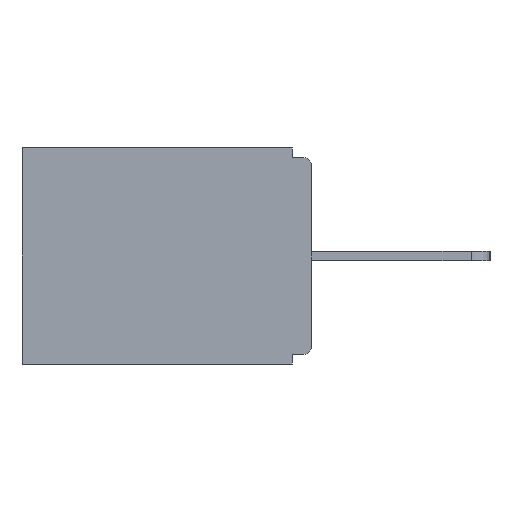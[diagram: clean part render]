
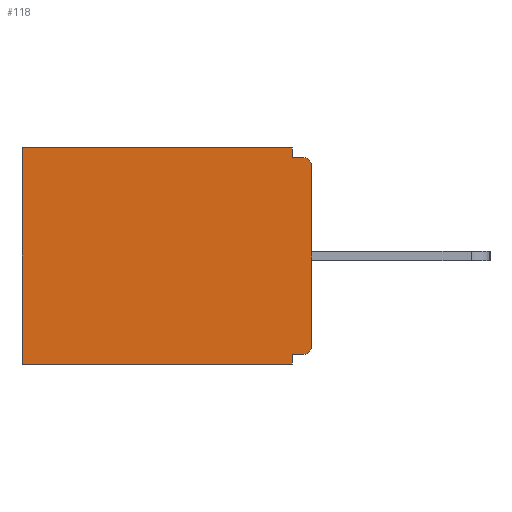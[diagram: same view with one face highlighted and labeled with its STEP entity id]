
A CAD part, left-side view. The second image highlights one B-rep face of the part: STEP entity #118.
In plain terms, the highlighted planar face has unit normal (-1, 0, 0).
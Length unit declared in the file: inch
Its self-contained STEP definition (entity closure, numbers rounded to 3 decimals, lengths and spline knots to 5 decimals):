
#29 = ORIENTED_EDGE ( 'NONE', *, *, #69, .F. ) ;
#69 = EDGE_CURVE ( 'NONE', #5602, #6535, #3409, .T. ) ;
#118 = ADVANCED_FACE ( 'NONE', ( #5495 ), #9830, .F. ) ;
#1013 = CARTESIAN_POINT ( 'NONE',  ( 0.298, 0.031, -0.343 ) ) ;
#1296 = VERTEX_POINT ( 'NONE', #2700 ) ;
#1427 = ORIENTED_EDGE ( 'NONE', *, *, #3058, .F. ) ;
#1451 = VERTEX_POINT ( 'NONE', #1707 ) ;
#1529 = ORIENTED_EDGE ( 'NONE', *, *, #13600, .T. ) ;
#1683 = CIRCLE ( 'NONE', #3444, 0.015 ) ;
#1707 = CARTESIAN_POINT ( 'NONE',  ( 0.298, 0.031, -0.343 ) ) ;
#1719 = VECTOR ( 'NONE', #12653, 39.37008 ) ;
#1757 = CARTESIAN_POINT ( 'NONE',  ( 0.298, 0.031, 0. ) ) ;
#1903 = VECTOR ( 'NONE', #17401, 39.37008 ) ;
#2360 = EDGE_CURVE ( 'NONE', #8241, #4948, #3593, .T. ) ;
#2376 = LINE ( 'NONE', #17199, #6337 ) ;
#2412 = LINE ( 'NONE', #14303, #10212 ) ;
#2489 = ORIENTED_EDGE ( 'NONE', *, *, #14761, .F. ) ;
#2700 = CARTESIAN_POINT ( 'NONE',  ( 0.298, 0.46, 0. ) ) ;
#2850 = CARTESIAN_POINT ( 'NONE',  ( 0.298, 0.015, -0.015 ) ) ;
#2875 = EDGE_CURVE ( 'NONE', #5602, #15154, #1683, .T. ) ;
#2887 = DIRECTION ( 'NONE',  ( 0., 0., -1. ) ) ;
#3058 = EDGE_CURVE ( 'NONE', #7864, #7671, #2376, .T. ) ;
#3164 = CARTESIAN_POINT ( 'NONE',  ( 0.298, 0., 0. ) ) ;
#3295 = CARTESIAN_POINT ( 'NONE',  ( 0.298, 0., 0. ) ) ;
#3409 = LINE ( 'NONE', #9230, #13443 ) ;
#3413 = EDGE_LOOP ( 'NONE', ( #5594, #10567, #1427, #1529, #5891, #2489, #17662, #15409, #12794, #29 ) ) ;
#3444 = AXIS2_PLACEMENT_3D ( 'NONE', #6610, #6570, #6550 ) ;
#3593 = LINE ( 'NONE', #6092, #17452 ) ;
#3798 = DIRECTION ( 'NONE',  ( 1., 0., 0. ) ) ;
#3959 = DIRECTION ( 'NONE',  ( 0., 1., 0. ) ) ;
#4643 = CARTESIAN_POINT ( 'NONE',  ( 0.298, 0.46, -0.343 ) ) ;
#4800 = DIRECTION ( 'NONE',  ( 0., 1., 0. ) ) ;
#4948 = VERTEX_POINT ( 'NONE', #13996 ) ;
#5204 = DIRECTION ( 'NONE',  ( 0., 0., -1. ) ) ;
#5298 = CARTESIAN_POINT ( 'NONE',  ( 0.298, 0., -0.03 ) ) ;
#5495 = FACE_OUTER_BOUND ( 'NONE', #3413, .T. ) ;
#5594 = ORIENTED_EDGE ( 'NONE', *, *, #2875, .T. ) ;
#5602 = VERTEX_POINT ( 'NONE', #5298 ) ;
#5680 = LINE ( 'NONE', #1013, #1719 ) ;
#5891 = ORIENTED_EDGE ( 'NONE', *, *, #10543, .T. ) ;
#6092 = CARTESIAN_POINT ( 'NONE',  ( 0.298, 0., -0.328 ) ) ;
#6204 = VERTEX_POINT ( 'NONE', #4643 ) ;
#6337 = VECTOR ( 'NONE', #14856, 39.37008 ) ;
#6535 = VERTEX_POINT ( 'NONE', #14258 ) ;
#6550 = DIRECTION ( 'NONE',  ( 0., 0., -1. ) ) ;
#6570 = DIRECTION ( 'NONE',  ( -1., 0., 0. ) ) ;
#6610 = CARTESIAN_POINT ( 'NONE',  ( 0.298, 0.015, -0.03 ) ) ;
#7373 = DIRECTION ( 'NONE',  ( 0., -1., 0. ) ) ;
#7671 = VERTEX_POINT ( 'NONE', #17305 ) ;
#7864 = VERTEX_POINT ( 'NONE', #1757 ) ;
#7906 = CARTESIAN_POINT ( 'NONE',  ( 0.298, 0., -0.343 ) ) ;
#8040 = LINE ( 'NONE', #9555, #11451 ) ;
#8241 = VERTEX_POINT ( 'NONE', #14052 ) ;
#9121 = EDGE_CURVE ( 'NONE', #8241, #6535, #12756, .T. ) ;
#9230 = CARTESIAN_POINT ( 'NONE',  ( 0.298, 0., 0. ) ) ;
#9555 = CARTESIAN_POINT ( 'NONE',  ( 0.298, 0.46, 0. ) ) ;
#9830 = PLANE ( 'NONE',  #15934 ) ;
#10212 = VECTOR ( 'NONE', #7373, 39.37008 ) ;
#10543 = EDGE_CURVE ( 'NONE', #1296, #6204, #8040, .T. ) ;
#10567 = ORIENTED_EDGE ( 'NONE', *, *, #17330, .F. ) ;
#11451 = VECTOR ( 'NONE', #5204, 39.37008 ) ;
#12653 = DIRECTION ( 'NONE',  ( 0., 0., -1. ) ) ;
#12756 = CIRCLE ( 'NONE', #14075, 0.015 ) ;
#12794 = ORIENTED_EDGE ( 'NONE', *, *, #9121, .T. ) ;
#12955 = LINE ( 'NONE', #7906, #1903 ) ;
#13443 = VECTOR ( 'NONE', #15652, 39.37008 ) ;
#13600 = EDGE_CURVE ( 'NONE', #7864, #1296, #18027, .T. ) ;
#13996 = CARTESIAN_POINT ( 'NONE',  ( 0.298, 0.031, -0.328 ) ) ;
#14052 = CARTESIAN_POINT ( 'NONE',  ( 0.298, 0.015, -0.328 ) ) ;
#14075 = AXIS2_PLACEMENT_3D ( 'NONE', #15311, #16979, #16953 ) ;
#14258 = CARTESIAN_POINT ( 'NONE',  ( 0.298, 0., -0.313 ) ) ;
#14303 = CARTESIAN_POINT ( 'NONE',  ( 0.298, 0., -0.015 ) ) ;
#14595 = VECTOR ( 'NONE', #4800, 39.37008 ) ;
#14761 = EDGE_CURVE ( 'NONE', #1451, #6204, #12955, .T. ) ;
#14856 = DIRECTION ( 'NONE',  ( 0., 0., -1. ) ) ;
#15154 = VERTEX_POINT ( 'NONE', #2850 ) ;
#15311 = CARTESIAN_POINT ( 'NONE',  ( 0.298, 0.015, -0.313 ) ) ;
#15409 = ORIENTED_EDGE ( 'NONE', *, *, #2360, .F. ) ;
#15652 = DIRECTION ( 'NONE',  ( 0., 0., -1. ) ) ;
#15934 = AXIS2_PLACEMENT_3D ( 'NONE', #3164, #3798, #2887 ) ;
#16953 = DIRECTION ( 'NONE',  ( 0., 0., -1. ) ) ;
#16979 = DIRECTION ( 'NONE',  ( -1., 0., 0. ) ) ;
#17164 = EDGE_CURVE ( 'NONE', #4948, #1451, #5680, .T. ) ;
#17199 = CARTESIAN_POINT ( 'NONE',  ( 0.298, 0.031, -0.343 ) ) ;
#17305 = CARTESIAN_POINT ( 'NONE',  ( 0.298, 0.031, -0.015 ) ) ;
#17330 = EDGE_CURVE ( 'NONE', #7671, #15154, #2412, .T. ) ;
#17401 = DIRECTION ( 'NONE',  ( 0., 1., 0. ) ) ;
#17452 = VECTOR ( 'NONE', #3959, 39.37008 ) ;
#17662 = ORIENTED_EDGE ( 'NONE', *, *, #17164, .F. ) ;
#18027 = LINE ( 'NONE', #3295, #14595 ) ;
